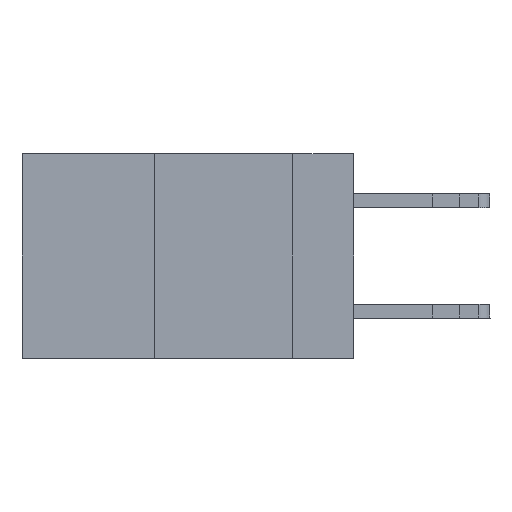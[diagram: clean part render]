
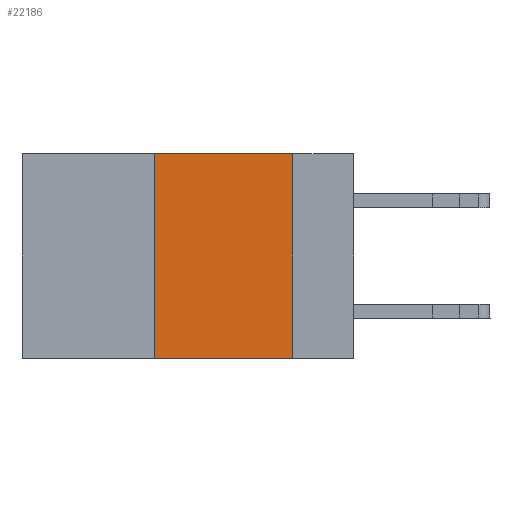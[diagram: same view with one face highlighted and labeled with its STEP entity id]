
A CAD part, left-side view. The second image highlights one B-rep face of the part: STEP entity #22186.
In plain terms, the highlighted planar face has unit normal (-1, 0, 0).
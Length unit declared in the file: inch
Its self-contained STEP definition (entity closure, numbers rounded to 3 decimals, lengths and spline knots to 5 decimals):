
#437 = FACE_OUTER_BOUND ( 'NONE', #15010, .T. ) ;
#2655 = LINE ( 'NONE', #12322, #12684 ) ;
#2792 = CARTESIAN_POINT ( 'NONE',  ( 0., 0.36, 0. ) ) ;
#2832 = LINE ( 'NONE', #24968, #8906 ) ;
#2922 = PLANE ( 'NONE',  #17420 ) ;
#3269 = VERTEX_POINT ( 'NONE', #24866 ) ;
#4318 = VERTEX_POINT ( 'NONE', #6075 ) ;
#5100 = DIRECTION ( 'NONE',  ( 0., 0., -1. ) ) ;
#6075 = CARTESIAN_POINT ( 'NONE',  ( 0., 0.11, 0. ) ) ;
#6345 = VECTOR ( 'NONE', #26814, 39.37008 ) ;
#7180 = CARTESIAN_POINT ( 'NONE',  ( 0., 0.6, 0. ) ) ;
#8906 = VECTOR ( 'NONE', #15431, 39.37008 ) ;
#9066 = ORIENTED_EDGE ( 'NONE', *, *, #10149, .T. ) ;
#10149 = EDGE_CURVE ( 'NONE', #3269, #25358, #2832, .T. ) ;
#10353 = EDGE_CURVE ( 'NONE', #4318, #25358, #26849, .T. ) ;
#11824 = CARTESIAN_POINT ( 'NONE',  ( 0., 0.36, 0. ) ) ;
#12322 = CARTESIAN_POINT ( 'NONE',  ( 0., 0.6, 0. ) ) ;
#12684 = VECTOR ( 'NONE', #14298, 39.37008 ) ;
#12882 = EDGE_CURVE ( 'NONE', #3269, #27393, #26394, .T. ) ;
#14298 = DIRECTION ( 'NONE',  ( 0., -1., 0. ) ) ;
#14408 = VECTOR ( 'NONE', #26005, 39.37008 ) ;
#15010 = EDGE_LOOP ( 'NONE', ( #22243, #23076, #24862, #9066 ) ) ;
#15431 = DIRECTION ( 'NONE',  ( 0., -1., 0. ) ) ;
#17420 = AXIS2_PLACEMENT_3D ( 'NONE', #7180, #24302, #5100 ) ;
#22186 = ADVANCED_FACE ( 'NONE', ( #437 ), #2922, .F. ) ;
#22243 = ORIENTED_EDGE ( 'NONE', *, *, #10353, .F. ) ;
#23076 = ORIENTED_EDGE ( 'NONE', *, *, #26057, .F. ) ;
#23591 = CARTESIAN_POINT ( 'NONE',  ( 0., 0.11, -0.37 ) ) ;
#23708 = CARTESIAN_POINT ( 'NONE',  ( 0., 0.11, 0. ) ) ;
#24302 = DIRECTION ( 'NONE',  ( 1., 0., 0. ) ) ;
#24862 = ORIENTED_EDGE ( 'NONE', *, *, #12882, .F. ) ;
#24866 = CARTESIAN_POINT ( 'NONE',  ( 0., 0.36, -0.37 ) ) ;
#24968 = CARTESIAN_POINT ( 'NONE',  ( 0., 0.6, -0.37 ) ) ;
#25358 = VERTEX_POINT ( 'NONE', #23591 ) ;
#26005 = DIRECTION ( 'NONE',  ( 0., 0., -1. ) ) ;
#26057 = EDGE_CURVE ( 'NONE', #27393, #4318, #2655, .T. ) ;
#26394 = LINE ( 'NONE', #11824, #6345 ) ;
#26814 = DIRECTION ( 'NONE',  ( 0., 0., 1. ) ) ;
#26849 = LINE ( 'NONE', #23708, #14408 ) ;
#27393 = VERTEX_POINT ( 'NONE', #2792 ) ;
